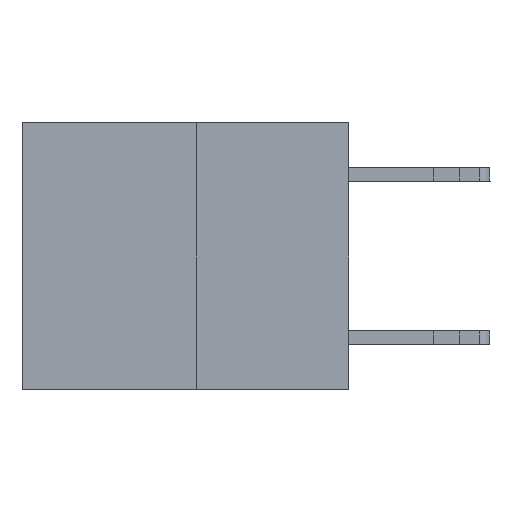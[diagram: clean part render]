
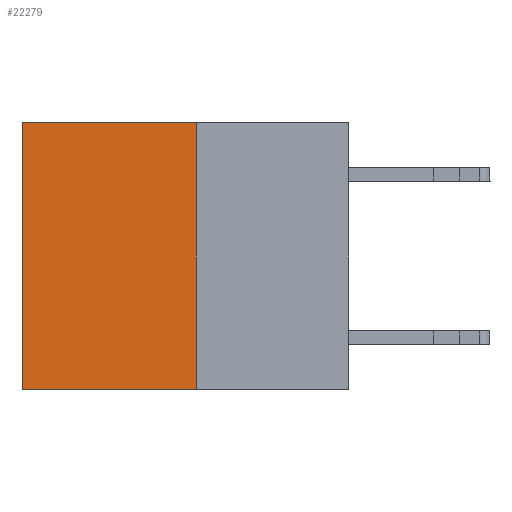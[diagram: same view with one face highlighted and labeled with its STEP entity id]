
A CAD part, left-side view. The second image highlights one B-rep face of the part: STEP entity #22279.
In plain terms, the highlighted planar face has unit normal (-1, 0, 0).
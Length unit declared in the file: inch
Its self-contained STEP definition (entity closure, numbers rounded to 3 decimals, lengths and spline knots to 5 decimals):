
#1893 = CARTESIAN_POINT ( 'NONE',  ( 0.3165, 0.28, -0.49 ) ) ;
#2739 = VERTEX_POINT ( 'NONE', #26608 ) ;
#4092 = ORIENTED_EDGE ( 'NONE', *, *, #19866, .T. ) ;
#4411 = AXIS2_PLACEMENT_3D ( 'NONE', #7253, #13883, #5052 ) ;
#4715 = DIRECTION ( 'NONE',  ( 0., 1., 0. ) ) ;
#5052 = DIRECTION ( 'NONE',  ( 0., 0., -1. ) ) ;
#5981 = VERTEX_POINT ( 'NONE', #10220 ) ;
#6063 = ORIENTED_EDGE ( 'NONE', *, *, #23858, .F. ) ;
#6340 = LINE ( 'NONE', #20629, #20805 ) ;
#6446 = EDGE_CURVE ( 'NONE', #5981, #23848, #7714, .T. ) ;
#6573 = LINE ( 'NONE', #17902, #11027 ) ;
#6962 = EDGE_CURVE ( 'NONE', #2739, #10817, #6340, .T. ) ;
#7253 = CARTESIAN_POINT ( 'NONE',  ( 0.3165, 0.28, -0.49 ) ) ;
#7525 = DIRECTION ( 'NONE',  ( 0., 0., -1. ) ) ;
#7714 = LINE ( 'NONE', #16280, #25008 ) ;
#7725 = LINE ( 'NONE', #16398, #23974 ) ;
#9476 = PLANE ( 'NONE',  #4411 ) ;
#10070 = ORIENTED_EDGE ( 'NONE', *, *, #6962, .F. ) ;
#10220 = CARTESIAN_POINT ( 'NONE',  ( 0.3165, 0.6, 0. ) ) ;
#10817 = VERTEX_POINT ( 'NONE', #1893 ) ;
#11027 = VECTOR ( 'NONE', #4715, 39.37008 ) ;
#11970 = DIRECTION ( 'NONE',  ( 0., 1., 0. ) ) ;
#13883 = DIRECTION ( 'NONE',  ( 1., 0., 0. ) ) ;
#16280 = CARTESIAN_POINT ( 'NONE',  ( 0.3165, 0.6, -0.49 ) ) ;
#16398 = CARTESIAN_POINT ( 'NONE',  ( 0.3165, 0.28, -0.49 ) ) ;
#17902 = CARTESIAN_POINT ( 'NONE',  ( 0.3165, 0.28, 0. ) ) ;
#19866 = EDGE_CURVE ( 'NONE', #2739, #5981, #6573, .T. ) ;
#20629 = CARTESIAN_POINT ( 'NONE',  ( 0.3165, 0.28, -0.49 ) ) ;
#20805 = VECTOR ( 'NONE', #22287, 39.37008 ) ;
#22279 = ADVANCED_FACE ( 'NONE', ( #25796 ), #9476, .F. ) ;
#22287 = DIRECTION ( 'NONE',  ( 0., 0., -1. ) ) ;
#22610 = CARTESIAN_POINT ( 'NONE',  ( 0.3165, 0.6, -0.49 ) ) ;
#23848 = VERTEX_POINT ( 'NONE', #22610 ) ;
#23858 = EDGE_CURVE ( 'NONE', #10817, #23848, #7725, .T. ) ;
#23974 = VECTOR ( 'NONE', #11970, 39.37008 ) ;
#24628 = EDGE_LOOP ( 'NONE', ( #27894, #6063, #10070, #4092 ) ) ;
#25008 = VECTOR ( 'NONE', #7525, 39.37008 ) ;
#25796 = FACE_OUTER_BOUND ( 'NONE', #24628, .T. ) ;
#26608 = CARTESIAN_POINT ( 'NONE',  ( 0.3165, 0.28, 0. ) ) ;
#27894 = ORIENTED_EDGE ( 'NONE', *, *, #6446, .T. ) ;
